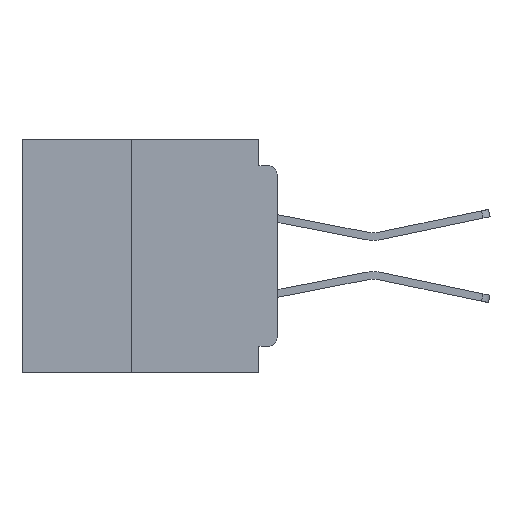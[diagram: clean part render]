
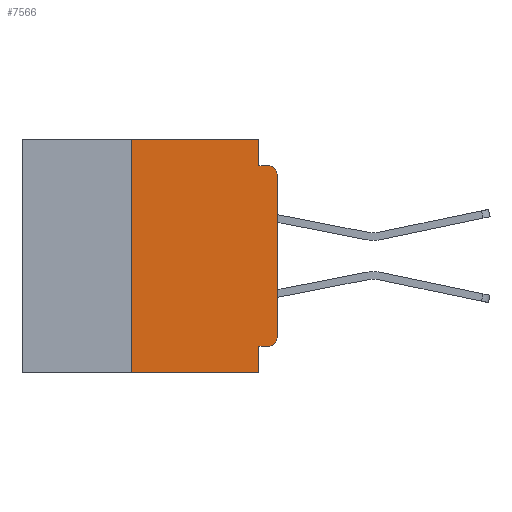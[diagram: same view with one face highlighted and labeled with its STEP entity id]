
A CAD part, left-side view. The second image highlights one B-rep face of the part: STEP entity #7566.
In plain terms, the highlighted planar face has unit normal (-1, 0, 0).
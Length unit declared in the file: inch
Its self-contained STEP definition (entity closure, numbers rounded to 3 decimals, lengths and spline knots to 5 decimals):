
#723 = EDGE_CURVE ( 'NONE', #46713, #57519, #54999, .T. ) ;
#732 = CARTESIAN_POINT ( 'NONE',  ( 0., 0.25, 0. ) ) ;
#2043 = VERTEX_POINT ( 'NONE', #27927 ) ;
#2410 = CIRCLE ( 'NONE', #11734, 0.015 ) ;
#2807 = AXIS2_PLACEMENT_3D ( 'NONE', #17521, #49692, #22166 ) ;
#3205 = EDGE_CURVE ( 'NONE', #28775, #46186, #39844, .T. ) ;
#3401 = CARTESIAN_POINT ( 'NONE',  ( 0., 0.25, -0.4 ) ) ;
#4351 = VERTEX_POINT ( 'NONE', #8230 ) ;
#4719 = DIRECTION ( 'NONE',  ( 0., -1., 0. ) ) ;
#5675 = ORIENTED_EDGE ( 'NONE', *, *, #36416, .T. ) ;
#7459 = DIRECTION ( 'NONE',  ( 0., 0., 1. ) ) ;
#7566 = ADVANCED_FACE ( 'NONE', ( #17761 ), #32791, .F. ) ;
#8230 = CARTESIAN_POINT ( 'NONE',  ( 0., 0., -0.34 ) ) ;
#10516 = DIRECTION ( 'NONE',  ( 0., 0., -1. ) ) ;
#11734 = AXIS2_PLACEMENT_3D ( 'NONE', #39266, #11768, #43921 ) ;
#11768 = DIRECTION ( 'NONE',  ( -1., 0., 0. ) ) ;
#12993 = CARTESIAN_POINT ( 'NONE',  ( 0., 0.031, 0. ) ) ;
#13248 = VECTOR ( 'NONE', #25225, 39.37008 ) ;
#13789 = ORIENTED_EDGE ( 'NONE', *, *, #45355, .T. ) ;
#15537 = CARTESIAN_POINT ( 'NONE',  ( 0., 0.015, -0.045 ) ) ;
#15694 = VERTEX_POINT ( 'NONE', #48884 ) ;
#17521 = CARTESIAN_POINT ( 'NONE',  ( 0., 0.015, -0.06 ) ) ;
#17761 = FACE_OUTER_BOUND ( 'NONE', #22755, .T. ) ;
#19169 = CARTESIAN_POINT ( 'NONE',  ( 0., 0.437, 0. ) ) ;
#21057 = LINE ( 'NONE', #3401, #23931 ) ;
#21782 = CARTESIAN_POINT ( 'NONE',  ( 0., 0.437, -0.4 ) ) ;
#22166 = DIRECTION ( 'NONE',  ( 0., 0., -1. ) ) ;
#22755 = EDGE_LOOP ( 'NONE', ( #46084, #13789, #51076, #53729, #29420, #59709, #25469, #38476, #27045, #5675 ) ) ;
#23063 = CARTESIAN_POINT ( 'NONE',  ( 0., 0.437, 0. ) ) ;
#23231 = DIRECTION ( 'NONE',  ( 0., 0., -1. ) ) ;
#23791 = DIRECTION ( 'NONE',  ( 0., 0., -1. ) ) ;
#23931 = VECTOR ( 'NONE', #35577, 39.37008 ) ;
#25225 = DIRECTION ( 'NONE',  ( 0., -1., 0. ) ) ;
#25469 = ORIENTED_EDGE ( 'NONE', *, *, #59428, .T. ) ;
#25812 = VECTOR ( 'NONE', #53880, 39.37008 ) ;
#27045 = ORIENTED_EDGE ( 'NONE', *, *, #723, .F. ) ;
#27619 = VECTOR ( 'NONE', #4719, 39.37008 ) ;
#27927 = CARTESIAN_POINT ( 'NONE',  ( 0., 0.031, -0.4 ) ) ;
#28775 = VERTEX_POINT ( 'NONE', #732 ) ;
#29420 = ORIENTED_EDGE ( 'NONE', *, *, #3205, .F. ) ;
#30356 = CARTESIAN_POINT ( 'NONE',  ( 0., 0., 0. ) ) ;
#32791 = PLANE ( 'NONE',  #54455 ) ;
#33353 = CARTESIAN_POINT ( 'NONE',  ( 0., 0., -0.06 ) ) ;
#34067 = VERTEX_POINT ( 'NONE', #58644 ) ;
#34586 = CARTESIAN_POINT ( 'NONE',  ( 0., 0.031, -0.355 ) ) ;
#34990 = EDGE_CURVE ( 'NONE', #57519, #2043, #43643, .T. ) ;
#35577 = DIRECTION ( 'NONE',  ( 0., 0., 1. ) ) ;
#36376 = EDGE_CURVE ( 'NONE', #34067, #41141, #48517, .T. ) ;
#36416 = EDGE_CURVE ( 'NONE', #46713, #4351, #2410, .T. ) ;
#38011 = CARTESIAN_POINT ( 'NONE',  ( 0., 0.031, -0.4 ) ) ;
#38383 = CIRCLE ( 'NONE', #2807, 0.015 ) ;
#38476 = ORIENTED_EDGE ( 'NONE', *, *, #34990, .F. ) ;
#39045 = DIRECTION ( 'NONE',  ( 0., 1., 0. ) ) ;
#39266 = CARTESIAN_POINT ( 'NONE',  ( 0., 0.015, -0.34 ) ) ;
#39296 = CARTESIAN_POINT ( 'NONE',  ( 0., 0., -0.355 ) ) ;
#39844 = LINE ( 'NONE', #23063, #27619 ) ;
#41141 = VERTEX_POINT ( 'NONE', #15537 ) ;
#41359 = VECTOR ( 'NONE', #39045, 39.37008 ) ;
#43385 = VECTOR ( 'NONE', #7459, 39.37008 ) ;
#43643 = LINE ( 'NONE', #38011, #45106 ) ;
#43921 = DIRECTION ( 'NONE',  ( 0., 0., -1. ) ) ;
#44854 = EDGE_CURVE ( 'NONE', #46186, #34067, #50430, .T. ) ;
#44863 = LINE ( 'NONE', #30356, #43385 ) ;
#45106 = VECTOR ( 'NONE', #10516, 39.37008 ) ;
#45355 = EDGE_CURVE ( 'NONE', #57848, #41141, #38383, .T. ) ;
#46084 = ORIENTED_EDGE ( 'NONE', *, *, #56875, .T. ) ;
#46186 = VERTEX_POINT ( 'NONE', #12993 ) ;
#46713 = VERTEX_POINT ( 'NONE', #58117 ) ;
#48018 = CARTESIAN_POINT ( 'NONE',  ( 0., 0.031, 0. ) ) ;
#48517 = LINE ( 'NONE', #52748, #13248 ) ;
#48884 = CARTESIAN_POINT ( 'NONE',  ( 0., 0.25, -0.4 ) ) ;
#49692 = DIRECTION ( 'NONE',  ( -1., 0., 0. ) ) ;
#50430 = LINE ( 'NONE', #48018, #51495 ) ;
#51076 = ORIENTED_EDGE ( 'NONE', *, *, #36376, .F. ) ;
#51293 = DIRECTION ( 'NONE',  ( 1., 0., 0. ) ) ;
#51495 = VECTOR ( 'NONE', #23231, 39.37008 ) ;
#51693 = LINE ( 'NONE', #21782, #25812 ) ;
#52748 = CARTESIAN_POINT ( 'NONE',  ( 0., 0., -0.045 ) ) ;
#53729 = ORIENTED_EDGE ( 'NONE', *, *, #44854, .F. ) ;
#53880 = DIRECTION ( 'NONE',  ( 0., -1., 0. ) ) ;
#54455 = AXIS2_PLACEMENT_3D ( 'NONE', #19169, #51293, #23791 ) ;
#54999 = LINE ( 'NONE', #39296, #41359 ) ;
#56875 = EDGE_CURVE ( 'NONE', #4351, #57848, #44863, .T. ) ;
#57519 = VERTEX_POINT ( 'NONE', #34586 ) ;
#57645 = EDGE_CURVE ( 'NONE', #15694, #28775, #21057, .T. ) ;
#57848 = VERTEX_POINT ( 'NONE', #33353 ) ;
#58117 = CARTESIAN_POINT ( 'NONE',  ( 0., 0.015, -0.355 ) ) ;
#58644 = CARTESIAN_POINT ( 'NONE',  ( 0., 0.031, -0.045 ) ) ;
#59428 = EDGE_CURVE ( 'NONE', #15694, #2043, #51693, .T. ) ;
#59709 = ORIENTED_EDGE ( 'NONE', *, *, #57645, .F. ) ;
